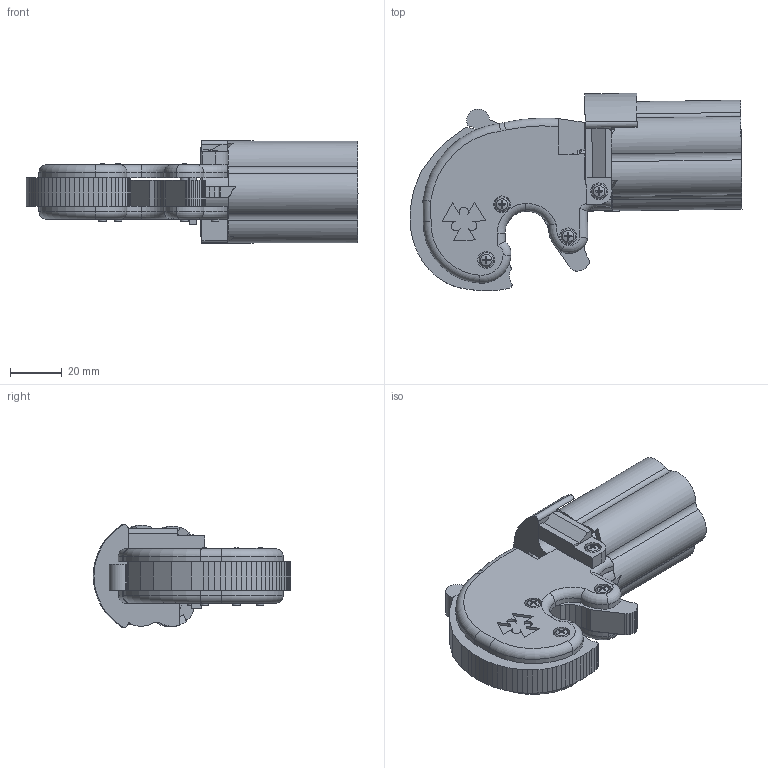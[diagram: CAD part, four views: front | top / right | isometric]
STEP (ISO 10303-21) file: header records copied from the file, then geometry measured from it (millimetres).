
FILE_DESCRIPTION((''),'2;1');
FILE_NAME('hexen.stp','2013-08-15T20:07:02',('mrfr'),(''),'Autodesk Inventor 2013','Autodesk Inventor 2013','');
FILE_SCHEMA(('AUTOMOTIVE_DESIGN { 1 0 10303 214 1 1 1 1 }'));
Length unit declared in the file: millimetre
Products named in the file (22): hexen; frame_R; cover; barrel; hammer; tube; trigger; frame_L; part; safe; lock; Šroubový spoj; ISO 7045 H M3 x 20 - 4.8 - H; ISO 4035 M3; ISO 7045 H M3 x 25 - 4.8 - H; spring; Kovaný šroub s hlavou s vnitřním vybráním - Metrický M3x0,5 x 60; Samojistná šestihranná matice - Ocel Metrický Property Class 5 and 10 - Metric M3 x 0.5 Typ kovu
Assembly tree (31 placements, depth 3):
  hexen
    frame_R
    cover
    barrel
    hammer
    tube  x6
    trigger
    frame_L
    part
    safe
    lock
    Šroubový spoj
      ISO 7045 H M3 x 20 - 4.8 - H
      ISO 4035 M3
    Šroubový spoj
      ISO 7045 H M3 x 20 - 4.8 - H
      ISO 4035 M3
    Šroubový spoj
      ISO 7045 H M3 x 20 - 4.8 - H
      ISO 4035 M3
    Šroubový spoj
      ISO 7045 H M3 x 25 - 4.8 - H
      ISO 4035 M3
    spring
    Šroubový spoj
      Kovaný šroub s hlavou s vnitřním vybráním - Metrický M3x0,5 x 60
      Samojistná šestihranná matice - Ocel Metrický Property Class 5 and 10 - Metric M3 x 0.5 Typ kovu
Bounding box: 127.97 x 76.13 x 39.67 mm (x, y, z)
Volume: 115897.9 mm3; surface area: 65055.8 mm2
Topology: 26 solids, 26 shells, 845 faces, 2335 edges, 1652 vertices
Faces by surface type: plane 574, cylinder 122, cone 75, torus 44, bspline 26, sphere 4
Full cylindrical faces by diameter (mm): 2 x1, 2.459 x5, 2.729 x4, 3 x18, 4 x2, 4.675 x1, 5.5 x1, 6 x6, 6.5 x4, 8 x13
Entity records: 24779 total; most frequent: CARTESIAN_POINT 5204, ORIENTED_EDGE 3802, DIRECTION 3707, EDGE_CURVE 1901, VECTOR 1475, LINE 1475, VERTEX_POINT 1286, AXIS2_PLACEMENT_3D 1116
